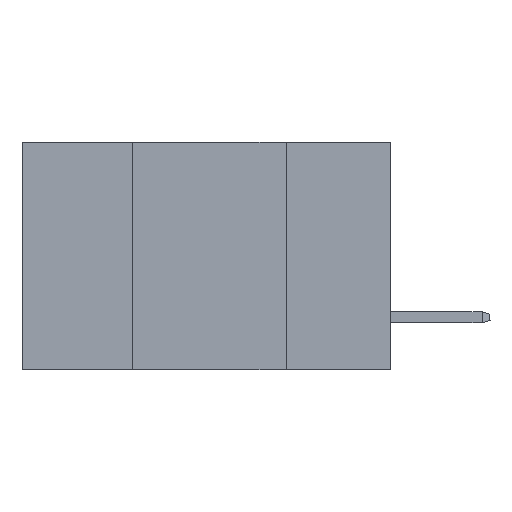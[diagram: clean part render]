
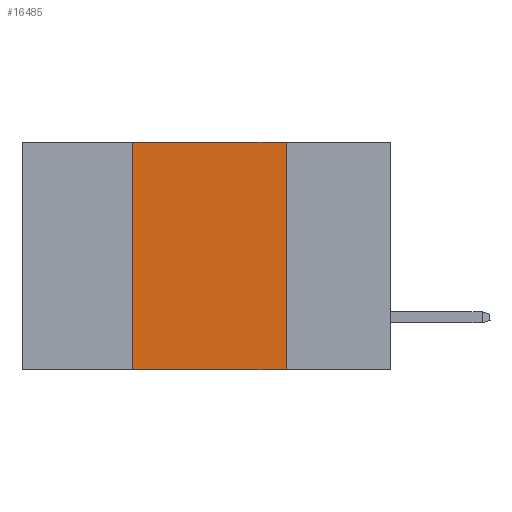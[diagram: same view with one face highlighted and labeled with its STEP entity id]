
A CAD part, left-side view. The second image highlights one B-rep face of the part: STEP entity #16485.
In plain terms, the highlighted planar face has unit normal (-1, 0, 0).
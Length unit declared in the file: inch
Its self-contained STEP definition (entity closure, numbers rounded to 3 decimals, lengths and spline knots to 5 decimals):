
#775 = CARTESIAN_POINT ( 'NONE',  ( 0., 0.6, 0. ) ) ;
#1225 = LINE ( 'NONE', #6370, #6453 ) ;
#1608 = CARTESIAN_POINT ( 'NONE',  ( 0., 0.17, -0.37 ) ) ;
#2632 = VERTEX_POINT ( 'NONE', #14805 ) ;
#3247 = EDGE_CURVE ( 'NONE', #19611, #7600, #10550, .T. ) ;
#4593 = VECTOR ( 'NONE', #7045, 39.37008 ) ;
#5470 = EDGE_CURVE ( 'NONE', #2632, #6165, #10455, .T. ) ;
#5776 = LINE ( 'NONE', #6714, #4593 ) ;
#5912 = CARTESIAN_POINT ( 'NONE',  ( 0., 0.6, -0.37 ) ) ;
#6165 = VERTEX_POINT ( 'NONE', #12277 ) ;
#6370 = CARTESIAN_POINT ( 'NONE',  ( 0., 0.17, 0. ) ) ;
#6453 = VECTOR ( 'NONE', #9900, 39.37008 ) ;
#6714 = CARTESIAN_POINT ( 'NONE',  ( 0., 0.42, 0. ) ) ;
#7045 = DIRECTION ( 'NONE',  ( 0., 0., 1. ) ) ;
#7600 = VERTEX_POINT ( 'NONE', #1608 ) ;
#7963 = CARTESIAN_POINT ( 'NONE',  ( 0., 0.42, -0.37 ) ) ;
#8248 = DIRECTION ( 'NONE',  ( 0., -1., 0. ) ) ;
#8561 = DIRECTION ( 'NONE',  ( 1., 0., 0. ) ) ;
#8857 = ORIENTED_EDGE ( 'NONE', *, *, #9352, .F. ) ;
#9352 = EDGE_CURVE ( 'NONE', #6165, #7600, #1225, .T. ) ;
#9900 = DIRECTION ( 'NONE',  ( 0., 0., -1. ) ) ;
#10455 = LINE ( 'NONE', #16043, #14293 ) ;
#10550 = LINE ( 'NONE', #5912, #11034 ) ;
#11034 = VECTOR ( 'NONE', #16796, 39.37008 ) ;
#11149 = FACE_OUTER_BOUND ( 'NONE', #17244, .T. ) ;
#12277 = CARTESIAN_POINT ( 'NONE',  ( 0., 0.17, 0. ) ) ;
#13098 = AXIS2_PLACEMENT_3D ( 'NONE', #775, #8561, #13487 ) ;
#13295 = PLANE ( 'NONE',  #13098 ) ;
#13487 = DIRECTION ( 'NONE',  ( 0., 0., -1. ) ) ;
#14209 = ORIENTED_EDGE ( 'NONE', *, *, #5470, .F. ) ;
#14293 = VECTOR ( 'NONE', #8248, 39.37008 ) ;
#14705 = ORIENTED_EDGE ( 'NONE', *, *, #15964, .F. ) ;
#14805 = CARTESIAN_POINT ( 'NONE',  ( 0., 0.42, 0. ) ) ;
#15964 = EDGE_CURVE ( 'NONE', #19611, #2632, #5776, .T. ) ;
#16043 = CARTESIAN_POINT ( 'NONE',  ( 0., 0.6, 0. ) ) ;
#16485 = ADVANCED_FACE ( 'NONE', ( #11149 ), #13295, .F. ) ;
#16796 = DIRECTION ( 'NONE',  ( 0., -1., 0. ) ) ;
#17244 = EDGE_LOOP ( 'NONE', ( #8857, #14209, #14705, #18620 ) ) ;
#18620 = ORIENTED_EDGE ( 'NONE', *, *, #3247, .T. ) ;
#19611 = VERTEX_POINT ( 'NONE', #7963 ) ;
